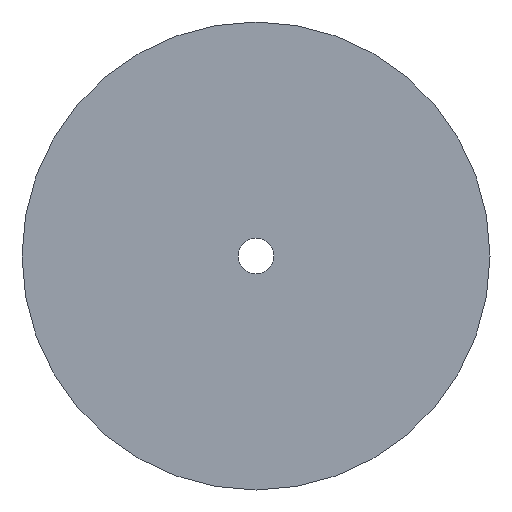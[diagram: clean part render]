
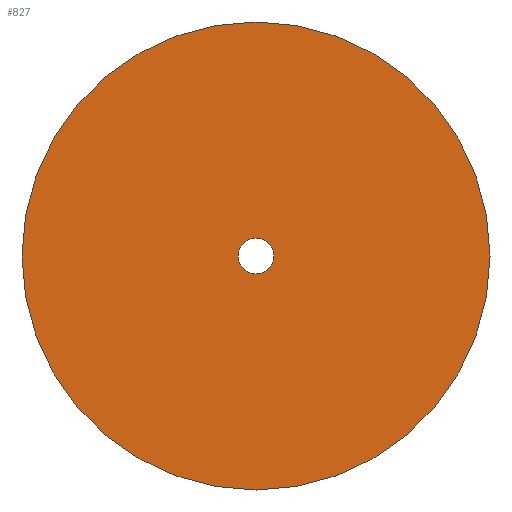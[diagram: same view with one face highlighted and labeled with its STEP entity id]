
A CAD part, front view. The second image highlights one B-rep face of the part: STEP entity #827.
In plain terms, the highlighted planar face has unit normal (0, -1, 0).
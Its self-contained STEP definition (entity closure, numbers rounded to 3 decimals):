
#192 = DIRECTION ( 'NONE',  ( 0., 0., -1. ) ) ;
#193 = DIRECTION ( 'NONE',  ( 0., -1., 0. ) ) ;
#203 = CARTESIAN_POINT ( 'NONE',  ( 0., 0.514, 0. ) ) ;
#210 = DIRECTION ( 'NONE',  ( 0., 0., -1. ) ) ;
#211 = DIRECTION ( 'NONE',  ( 0., -1., 0. ) ) ;
#221 = CARTESIAN_POINT ( 'NONE',  ( 0., 0.514, 0. ) ) ;
#284 = DIRECTION ( 'NONE',  ( 0., 0., -1. ) ) ;
#285 = DIRECTION ( 'NONE',  ( 0., -1., 0. ) ) ;
#286 = CARTESIAN_POINT ( 'NONE',  ( 2.5, 0.514, 0. ) ) ;
#287 = PLANE ( 'NONE',  #748 ) ;
#310 = DIRECTION ( 'NONE',  ( 0., 0., -1. ) ) ;
#311 = DIRECTION ( 'NONE',  ( 0., -1., 0. ) ) ;
#312 = CARTESIAN_POINT ( 'NONE',  ( 0., 0.514, 0. ) ) ;
#313 = DIRECTION ( 'NONE',  ( 0., 0., -1. ) ) ;
#314 = DIRECTION ( 'NONE',  ( 0., -1., 0. ) ) ;
#318 = CARTESIAN_POINT ( 'NONE',  ( 0., 0.514, 0. ) ) ;
#391 = CARTESIAN_POINT ( 'NONE',  ( 0., 0.514, 33. ) ) ;
#392 = CARTESIAN_POINT ( 'NONE',  ( 0., 0.514, -33. ) ) ;
#396 = CARTESIAN_POINT ( 'NONE',  ( 0., 0.514, 2.5 ) ) ;
#401 = CARTESIAN_POINT ( 'NONE',  ( 0., 0.514, -2.5 ) ) ;
#473 = VERTEX_POINT ( 'NONE', #401 ) ;
#478 = VERTEX_POINT ( 'NONE', #396 ) ;
#482 = VERTEX_POINT ( 'NONE', #392 ) ;
#483 = VERTEX_POINT ( 'NONE', #391 ) ;
#516 = EDGE_LOOP ( 'NONE', ( #621, #623 ) ) ;
#518 = EDGE_LOOP ( 'NONE', ( #619, #620 ) ) ;
#619 = ORIENTED_EDGE ( 'NONE', *, *, #846, .T. ) ;
#620 = ORIENTED_EDGE ( 'NONE', *, *, #791, .T. ) ;
#621 = ORIENTED_EDGE ( 'NONE', *, *, #792, .F. ) ;
#623 = ORIENTED_EDGE ( 'NONE', *, *, #851, .F. ) ;
#650 = AXIS2_PLACEMENT_3D ( 'NONE', #318, #314, #313 ) ;
#681 = AXIS2_PLACEMENT_3D ( 'NONE', #312, #311, #310 ) ;
#731 = AXIS2_PLACEMENT_3D ( 'NONE', #203, #193, #192 ) ;
#736 = AXIS2_PLACEMENT_3D ( 'NONE', #221, #211, #210 ) ;
#739 = FACE_OUTER_BOUND ( 'NONE', #518, .T. ) ;
#748 = AXIS2_PLACEMENT_3D ( 'NONE', #286, #285, #284 ) ;
#753 = FACE_BOUND ( 'NONE', #516, .T. ) ;
#791 = EDGE_CURVE ( 'NONE', #483, #482, #815, .T. ) ;
#792 = EDGE_CURVE ( 'NONE', #473, #478, #813, .T. ) ;
#808 = CIRCLE ( 'NONE', #731, 2.5 ) ;
#812 = CIRCLE ( 'NONE', #736, 33. ) ;
#813 = CIRCLE ( 'NONE', #681, 2.5 ) ;
#815 = CIRCLE ( 'NONE', #650, 33. ) ;
#827 = ADVANCED_FACE ( 'NONE', ( #739, #753 ), #287, .T. ) ;
#846 = EDGE_CURVE ( 'NONE', #482, #483, #812, .T. ) ;
#851 = EDGE_CURVE ( 'NONE', #478, #473, #808, .T. ) ;
